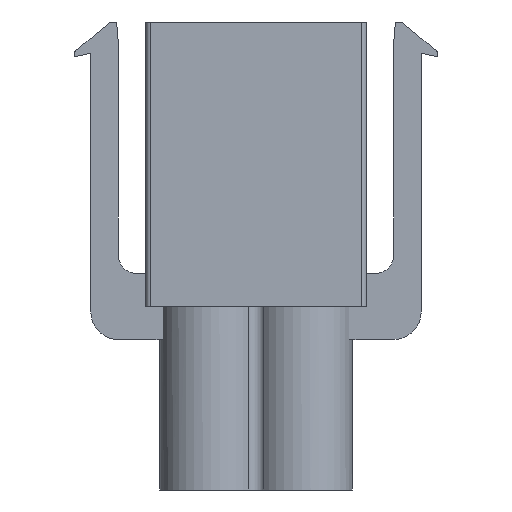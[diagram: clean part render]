
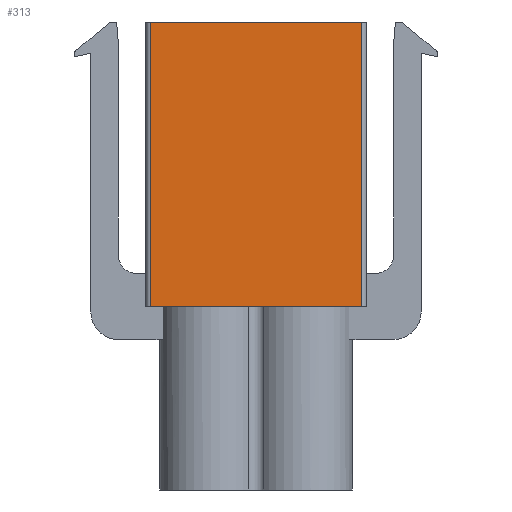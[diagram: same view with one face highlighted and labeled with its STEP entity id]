
A CAD part, front view. The second image highlights one B-rep face of the part: STEP entity #313.
In plain terms, the highlighted planar face has unit normal (0, -1, 0).
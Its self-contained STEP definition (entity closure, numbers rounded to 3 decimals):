
#186 = CARTESIAN_POINT ( 'NONE',  ( -5.75, -4.05, -15.5 ) ) ;
#291 = CARTESIAN_POINT ( 'NONE',  ( -5.75, -4.05, 0. ) ) ;
#313 = ADVANCED_FACE ( 'NONE', ( #1982 ), #5633, .T. ) ;
#548 = VECTOR ( 'NONE', #5356, 1000. ) ;
#638 = CARTESIAN_POINT ( 'NONE',  ( -6., -4.05, -15.5 ) ) ;
#722 = VECTOR ( 'NONE', #1808, 1000. ) ;
#1367 = ORIENTED_EDGE ( 'NONE', *, *, #6044, .F. ) ;
#1808 = DIRECTION ( 'NONE',  ( 1., 0., 0. ) ) ;
#1970 = CARTESIAN_POINT ( 'NONE',  ( 5.75, -4.05, 0. ) ) ;
#1982 = FACE_OUTER_BOUND ( 'NONE', #2469, .T. ) ;
#1996 = DIRECTION ( 'NONE',  ( 0., 0., 1. ) ) ;
#2022 = ORIENTED_EDGE ( 'NONE', *, *, #3809, .T. ) ;
#2097 = AXIS2_PLACEMENT_3D ( 'NONE', #4643, #6717, #6749 ) ;
#2469 = EDGE_LOOP ( 'NONE', ( #1367, #2022, #6483, #4876 ) ) ;
#2513 = VERTEX_POINT ( 'NONE', #1970 ) ;
#2589 = CARTESIAN_POINT ( 'NONE',  ( -5.75, -4.05, -15.5 ) ) ;
#2930 = CARTESIAN_POINT ( 'NONE',  ( 5.75, -4.05, -15.5 ) ) ;
#3156 = VERTEX_POINT ( 'NONE', #3844 ) ;
#3162 = VERTEX_POINT ( 'NONE', #291 ) ;
#3229 = VECTOR ( 'NONE', #5242, 1000. ) ;
#3276 = CARTESIAN_POINT ( 'NONE',  ( -6., -4.05, 0. ) ) ;
#3809 = EDGE_CURVE ( 'NONE', #3162, #4704, #4639, .T. ) ;
#3844 = CARTESIAN_POINT ( 'NONE',  ( 5.75, -4.05, -15.5 ) ) ;
#3956 = EDGE_CURVE ( 'NONE', #4704, #3156, #4879, .T. ) ;
#3962 = LINE ( 'NONE', #3276, #548 ) ;
#4594 = LINE ( 'NONE', #2930, #4928 ) ;
#4639 = LINE ( 'NONE', #2589, #3229 ) ;
#4643 = CARTESIAN_POINT ( 'NONE',  ( -6., -4.05, -15.5 ) ) ;
#4704 = VERTEX_POINT ( 'NONE', #186 ) ;
#4876 = ORIENTED_EDGE ( 'NONE', *, *, #6540, .T. ) ;
#4879 = LINE ( 'NONE', #638, #722 ) ;
#4928 = VECTOR ( 'NONE', #1996, 1000. ) ;
#5242 = DIRECTION ( 'NONE',  ( 0., 0., -1. ) ) ;
#5356 = DIRECTION ( 'NONE',  ( 1., 0., 0. ) ) ;
#5633 = PLANE ( 'NONE',  #2097 ) ;
#6044 = EDGE_CURVE ( 'NONE', #3162, #2513, #3962, .T. ) ;
#6483 = ORIENTED_EDGE ( 'NONE', *, *, #3956, .T. ) ;
#6540 = EDGE_CURVE ( 'NONE', #3156, #2513, #4594, .T. ) ;
#6717 = DIRECTION ( 'NONE',  ( 0., -1., 0. ) ) ;
#6749 = DIRECTION ( 'NONE',  ( 0., 0., -1. ) ) ;
